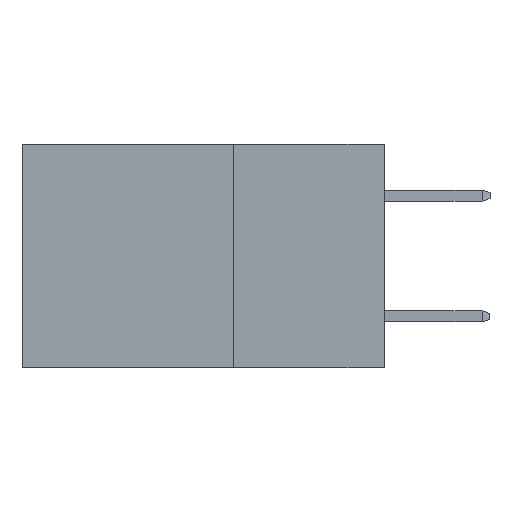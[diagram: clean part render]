
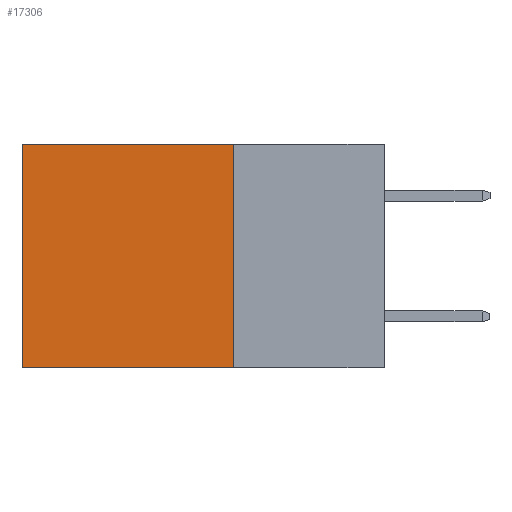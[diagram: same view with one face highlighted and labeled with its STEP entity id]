
A CAD part, left-side view. The second image highlights one B-rep face of the part: STEP entity #17306.
In plain terms, the highlighted planar face has unit normal (-1, 0, 0).
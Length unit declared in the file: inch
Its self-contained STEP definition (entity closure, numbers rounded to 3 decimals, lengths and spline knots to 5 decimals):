
#21 = VERTEX_POINT ( 'NONE', #16927 ) ;
#73 = CARTESIAN_POINT ( 'NONE',  ( 0.298, 0.25, -0.37 ) ) ;
#220 = CARTESIAN_POINT ( 'NONE',  ( 0.298, 0.25, 0. ) ) ;
#1349 = DIRECTION ( 'NONE',  ( 0., 0., -1. ) ) ;
#1610 = FACE_OUTER_BOUND ( 'NONE', #13427, .T. ) ;
#2634 = EDGE_CURVE ( 'NONE', #9362, #6837, #5031, .T. ) ;
#3200 = DIRECTION ( 'NONE',  ( 1., 0., 0. ) ) ;
#4351 = ORIENTED_EDGE ( 'NONE', *, *, #9803, .F. ) ;
#4970 = VECTOR ( 'NONE', #1349, 39.37008 ) ;
#5031 = LINE ( 'NONE', #5608, #9482 ) ;
#5608 = CARTESIAN_POINT ( 'NONE',  ( 0.298, 0.6, 0. ) ) ;
#5955 = LINE ( 'NONE', #11124, #17627 ) ;
#6395 = ORIENTED_EDGE ( 'NONE', *, *, #8712, .T. ) ;
#6837 = VERTEX_POINT ( 'NONE', #6916 ) ;
#6916 = CARTESIAN_POINT ( 'NONE',  ( 0.298, 0.6, -0.37 ) ) ;
#7561 = PLANE ( 'NONE',  #8658 ) ;
#7836 = EDGE_CURVE ( 'NONE', #21, #6837, #9040, .T. ) ;
#8658 = AXIS2_PLACEMENT_3D ( 'NONE', #220, #3200, #13489 ) ;
#8680 = ORIENTED_EDGE ( 'NONE', *, *, #7836, .F. ) ;
#8712 = EDGE_CURVE ( 'NONE', #10255, #9362, #5955, .T. ) ;
#9040 = LINE ( 'NONE', #73, #12474 ) ;
#9362 = VERTEX_POINT ( 'NONE', #12569 ) ;
#9482 = VECTOR ( 'NONE', #15870, 39.37008 ) ;
#9803 = EDGE_CURVE ( 'NONE', #10255, #21, #16671, .T. ) ;
#10255 = VERTEX_POINT ( 'NONE', #10376 ) ;
#10376 = CARTESIAN_POINT ( 'NONE',  ( 0.298, 0.25, 0. ) ) ;
#11062 = DIRECTION ( 'NONE',  ( 0., 1., 0. ) ) ;
#11124 = CARTESIAN_POINT ( 'NONE',  ( 0.298, 0.25, 0. ) ) ;
#12474 = VECTOR ( 'NONE', #13295, 39.37008 ) ;
#12569 = CARTESIAN_POINT ( 'NONE',  ( 0.298, 0.6, 0. ) ) ;
#13295 = DIRECTION ( 'NONE',  ( 0., 1., 0. ) ) ;
#13427 = EDGE_LOOP ( 'NONE', ( #16465, #8680, #4351, #6395 ) ) ;
#13489 = DIRECTION ( 'NONE',  ( 0., 0., -1. ) ) ;
#15870 = DIRECTION ( 'NONE',  ( 0., 0., -1. ) ) ;
#16465 = ORIENTED_EDGE ( 'NONE', *, *, #2634, .T. ) ;
#16671 = LINE ( 'NONE', #18866, #4970 ) ;
#16927 = CARTESIAN_POINT ( 'NONE',  ( 0.298, 0.25, -0.37 ) ) ;
#17306 = ADVANCED_FACE ( 'NONE', ( #1610 ), #7561, .F. ) ;
#17627 = VECTOR ( 'NONE', #11062, 39.37008 ) ;
#18866 = CARTESIAN_POINT ( 'NONE',  ( 0.298, 0.25, 0. ) ) ;
